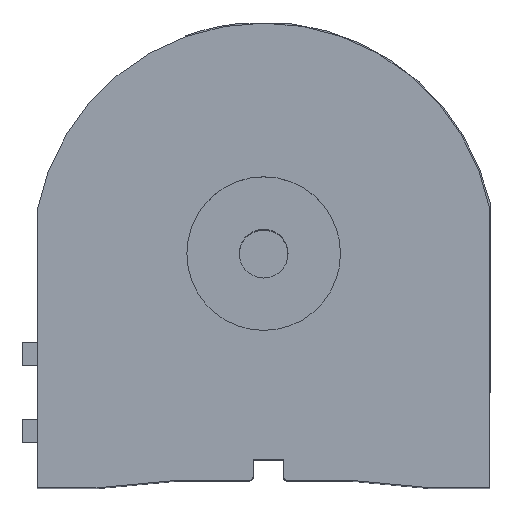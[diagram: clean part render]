
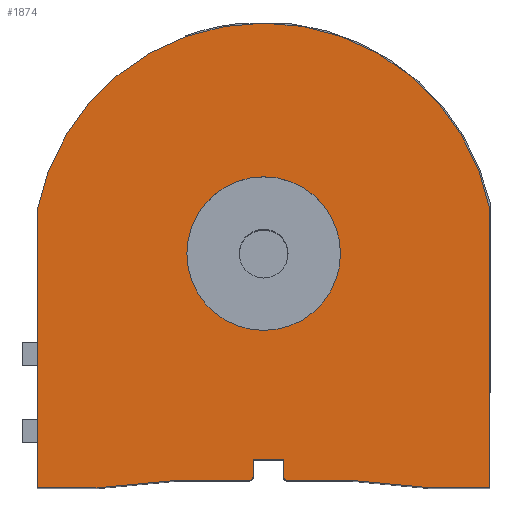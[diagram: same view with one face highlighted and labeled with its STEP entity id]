
A CAD part, top view. The second image highlights one B-rep face of the part: STEP entity #1874.
In plain terms, the highlighted planar face has unit normal (0, 0, 1).
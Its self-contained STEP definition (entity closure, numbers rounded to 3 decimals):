
#7 = CARTESIAN_POINT ( 'NONE',  ( -22.5, -59., 80. ) ) ;
#67 = ORIENTED_EDGE ( 'NONE', *, *, #3143, .F. ) ;
#74 = LINE ( 'NONE', #588, #1202 ) ;
#77 = ORIENTED_EDGE ( 'NONE', *, *, #887, .T. ) ;
#78 = LINE ( 'NONE', #2872, #2936 ) ;
#91 = EDGE_CURVE ( 'NONE', #2361, #855, #78, .T. ) ;
#120 = VERTEX_POINT ( 'NONE', #1077 ) ;
#165 = DIRECTION ( 'NONE',  ( 0., 0., 1. ) ) ;
#188 = LINE ( 'NONE', #1919, #3088 ) ;
#200 = FACE_OUTER_BOUND ( 'NONE', #2185, .T. ) ;
#226 = CARTESIAN_POINT ( 'NONE',  ( 5.083, -58., 80. ) ) ;
#251 = DIRECTION ( 'NONE',  ( -1., 0., 0. ) ) ;
#319 = VERTEX_POINT ( 'NONE', #458 ) ;
#347 = VECTOR ( 'NONE', #2061, 1000. ) ;
#356 = EDGE_CURVE ( 'NONE', #688, #815, #2359, .T. ) ;
#370 = CARTESIAN_POINT ( 'NONE',  ( -43.909, -61., 80. ) ) ;
#433 = EDGE_CURVE ( 'NONE', #1744, #2437, #3101, .T. ) ;
#435 = LINE ( 'NONE', #1690, #1250 ) ;
#446 = EDGE_CURVE ( 'NONE', #815, #3142, #2324, .T. ) ;
#458 = CARTESIAN_POINT ( 'NONE',  ( -3.75, -59., 80. ) ) ;
#480 = EDGE_LOOP ( 'NONE', ( #2577, #3135 ) ) ;
#489 = EDGE_CURVE ( 'NONE', #2361, #910, #1838, .T. ) ;
#490 = CARTESIAN_POINT ( 'NONE',  ( 0., 0., 80. ) ) ;
#495 = VERTEX_POINT ( 'NONE', #574 ) ;
#513 = EDGE_CURVE ( 'NONE', #1744, #714, #2102, .T. ) ;
#517 = EDGE_CURVE ( 'NONE', #855, #1277, #74, .T. ) ;
#518 = CIRCLE ( 'NONE', #3257, 20. ) ;
#574 = CARTESIAN_POINT ( 'NONE',  ( -20., 0., 80. ) ) ;
#588 = CARTESIAN_POINT ( 'NONE',  ( 5.083, -53.5, 80. ) ) ;
#611 = CIRCLE ( 'NONE', #2447, 20. ) ;
#667 = LINE ( 'NONE', #1197, #1941 ) ;
#688 = VERTEX_POINT ( 'NONE', #3011 ) ;
#714 = VERTEX_POINT ( 'NONE', #1204 ) ;
#741 = DIRECTION ( 'NONE',  ( 0., 0., 1. ) ) ;
#778 = VECTOR ( 'NONE', #1339, 1000. ) ;
#788 = ORIENTED_EDGE ( 'NONE', *, *, #489, .T. ) ;
#794 = EDGE_CURVE ( 'NONE', #2437, #688, #1452, .T. ) ;
#808 = LINE ( 'NONE', #1074, #2657 ) ;
#815 = VERTEX_POINT ( 'NONE', #3045 ) ;
#817 = CIRCLE ( 'NONE', #1404, 1. ) ;
#822 = CARTESIAN_POINT ( 'NONE',  ( -3.75, -58., 80. ) ) ;
#844 = CARTESIAN_POINT ( 'NONE',  ( -58.909, -61., 80. ) ) ;
#855 = VERTEX_POINT ( 'NONE', #2562 ) ;
#887 = EDGE_CURVE ( 'NONE', #319, #3008, #817, .T. ) ;
#910 = VERTEX_POINT ( 'NONE', #2580 ) ;
#1051 = CARTESIAN_POINT ( 'NONE',  ( -58.909, -61., 80. ) ) ;
#1074 = CARTESIAN_POINT ( 'NONE',  ( 58.909, -61., 80. ) ) ;
#1077 = CARTESIAN_POINT ( 'NONE',  ( 20., 0., 80. ) ) ;
#1078 = CARTESIAN_POINT ( 'NONE',  ( -2.75, -53.5, 80. ) ) ;
#1090 = AXIS2_PLACEMENT_3D ( 'NONE', #3216, #1494, #251 ) ;
#1092 = DIRECTION ( 'NONE',  ( -1., 0., 0. ) ) ;
#1179 = ORIENTED_EDGE ( 'NONE', *, *, #2942, .F. ) ;
#1197 = CARTESIAN_POINT ( 'NONE',  ( 22.5, -59., 80. ) ) ;
#1202 = VECTOR ( 'NONE', #1092, 1000. ) ;
#1204 = CARTESIAN_POINT ( 'NONE',  ( 22.5, -59., 80. ) ) ;
#1216 = ORIENTED_EDGE ( 'NONE', *, *, #91, .F. ) ;
#1240 = PLANE ( 'NONE',  #1090 ) ;
#1250 = VECTOR ( 'NONE', #2176, 1000. ) ;
#1256 = VECTOR ( 'NONE', #2119, 1000. ) ;
#1277 = VERTEX_POINT ( 'NONE', #1078 ) ;
#1280 = DIRECTION ( 'NONE',  ( 0., 0., 1. ) ) ;
#1339 = DIRECTION ( 'NONE',  ( -0.996, 0.093, 0. ) ) ;
#1404 = AXIS2_PLACEMENT_3D ( 'NONE', #822, #2810, #2596 ) ;
#1447 = DIRECTION ( 'NONE',  ( -1., 0., 0. ) ) ;
#1452 = LINE ( 'NONE', #2445, #2630 ) ;
#1494 = DIRECTION ( 'NONE',  ( 0., 0., -1. ) ) ;
#1612 = DIRECTION ( 'NONE',  ( 0., 1., 0. ) ) ;
#1636 = VECTOR ( 'NONE', #2067, 1000. ) ;
#1661 = EDGE_CURVE ( 'NONE', #3142, #1814, #808, .T. ) ;
#1688 = AXIS2_PLACEMENT_3D ( 'NONE', #490, #741, #2697 ) ;
#1690 = CARTESIAN_POINT ( 'NONE',  ( -2.75, -53.5, 80. ) ) ;
#1736 = CARTESIAN_POINT ( 'NONE',  ( 0., 0., 80. ) ) ;
#1744 = VERTEX_POINT ( 'NONE', #2656 ) ;
#1787 = AXIS2_PLACEMENT_3D ( 'NONE', #2835, #2338, #2049 ) ;
#1813 = EDGE_CURVE ( 'NONE', #495, #120, #518, .T. ) ;
#1814 = VERTEX_POINT ( 'NONE', #2435 ) ;
#1838 = CIRCLE ( 'NONE', #1787, 1. ) ;
#1874 = ADVANCED_FACE ( 'NONE', ( #1986, #200 ), #1240, .F. ) ;
#1919 = CARTESIAN_POINT ( 'NONE',  ( 22.5, -59., 80. ) ) ;
#1926 = ORIENTED_EDGE ( 'NONE', *, *, #794, .T. ) ;
#1941 = VECTOR ( 'NONE', #1447, 1000. ) ;
#1950 = DIRECTION ( 'NONE',  ( -1., 0., 0. ) ) ;
#1986 = FACE_BOUND ( 'NONE', #480, .T. ) ;
#1995 = CARTESIAN_POINT ( 'NONE',  ( -2.75, -58., 80. ) ) ;
#2049 = DIRECTION ( 'NONE',  ( -1., 0., 0. ) ) ;
#2061 = DIRECTION ( 'NONE',  ( -0.996, -0.093, 0. ) ) ;
#2067 = DIRECTION ( 'NONE',  ( 1., 0., 0. ) ) ;
#2075 = ORIENTED_EDGE ( 'NONE', *, *, #446, .T. ) ;
#2102 = LINE ( 'NONE', #2783, #778 ) ;
#2119 = DIRECTION ( 'NONE',  ( 0., -1., 0. ) ) ;
#2127 = LINE ( 'NONE', #370, #347 ) ;
#2176 = DIRECTION ( 'NONE',  ( 0., -1., 0. ) ) ;
#2185 = EDGE_LOOP ( 'NONE', ( #1216, #788, #3255, #2742, #2579, #1926, #2369, #2075, #2870, #67, #2809, #77, #1179, #2267 ) ) ;
#2267 = ORIENTED_EDGE ( 'NONE', *, *, #517, .F. ) ;
#2273 = CARTESIAN_POINT ( 'NONE',  ( 58.909, -61., 80. ) ) ;
#2324 = LINE ( 'NONE', #844, #1256 ) ;
#2338 = DIRECTION ( 'NONE',  ( 0., 0., 1. ) ) ;
#2359 = CIRCLE ( 'NONE', #1688, 60. ) ;
#2361 = VERTEX_POINT ( 'NONE', #226 ) ;
#2369 = ORIENTED_EDGE ( 'NONE', *, *, #356, .T. ) ;
#2422 = CARTESIAN_POINT ( 'NONE',  ( 0., 0., 80. ) ) ;
#2435 = CARTESIAN_POINT ( 'NONE',  ( -43.909, -61., 80. ) ) ;
#2437 = VERTEX_POINT ( 'NONE', #2273 ) ;
#2445 = CARTESIAN_POINT ( 'NONE',  ( 58.909, -61., 80. ) ) ;
#2447 = AXIS2_PLACEMENT_3D ( 'NONE', #1736, #1280, #2726 ) ;
#2535 = VERTEX_POINT ( 'NONE', #7 ) ;
#2562 = CARTESIAN_POINT ( 'NONE',  ( 5.083, -53.5, 80. ) ) ;
#2577 = ORIENTED_EDGE ( 'NONE', *, *, #3072, .F. ) ;
#2579 = ORIENTED_EDGE ( 'NONE', *, *, #433, .T. ) ;
#2580 = CARTESIAN_POINT ( 'NONE',  ( 6.083, -59., 80. ) ) ;
#2583 = CARTESIAN_POINT ( 'NONE',  ( 58.909, -61., 80. ) ) ;
#2596 = DIRECTION ( 'NONE',  ( -1., 0., 0. ) ) ;
#2630 = VECTOR ( 'NONE', #2710, 1000. ) ;
#2656 = CARTESIAN_POINT ( 'NONE',  ( 43.909, -61., 80. ) ) ;
#2657 = VECTOR ( 'NONE', #2836, 1000. ) ;
#2697 = DIRECTION ( 'NONE',  ( -1., 0., 0. ) ) ;
#2710 = DIRECTION ( 'NONE',  ( 0., 1., 0. ) ) ;
#2726 = DIRECTION ( 'NONE',  ( 1., 0., 0. ) ) ;
#2742 = ORIENTED_EDGE ( 'NONE', *, *, #513, .F. ) ;
#2783 = CARTESIAN_POINT ( 'NONE',  ( 43.909, -61., 80. ) ) ;
#2809 = ORIENTED_EDGE ( 'NONE', *, *, #3259, .F. ) ;
#2810 = DIRECTION ( 'NONE',  ( 0., 0., 1. ) ) ;
#2835 = CARTESIAN_POINT ( 'NONE',  ( 6.083, -58., 80. ) ) ;
#2836 = DIRECTION ( 'NONE',  ( 1., 0., 0. ) ) ;
#2870 = ORIENTED_EDGE ( 'NONE', *, *, #1661, .T. ) ;
#2872 = CARTESIAN_POINT ( 'NONE',  ( 5.083, -66.165, 80. ) ) ;
#2915 = EDGE_CURVE ( 'NONE', #714, #910, #188, .T. ) ;
#2936 = VECTOR ( 'NONE', #1612, 1000. ) ;
#2942 = EDGE_CURVE ( 'NONE', #1277, #3008, #435, .T. ) ;
#3008 = VERTEX_POINT ( 'NONE', #1995 ) ;
#3011 = CARTESIAN_POINT ( 'NONE',  ( 58.909, 11.39, 80. ) ) ;
#3045 = CARTESIAN_POINT ( 'NONE',  ( -58.909, 11.39, 80. ) ) ;
#3072 = EDGE_CURVE ( 'NONE', #120, #495, #611, .T. ) ;
#3088 = VECTOR ( 'NONE', #1950, 1000. ) ;
#3101 = LINE ( 'NONE', #2583, #1636 ) ;
#3135 = ORIENTED_EDGE ( 'NONE', *, *, #1813, .F. ) ;
#3142 = VERTEX_POINT ( 'NONE', #1051 ) ;
#3143 = EDGE_CURVE ( 'NONE', #2535, #1814, #2127, .T. ) ;
#3202 = DIRECTION ( 'NONE',  ( 1., 0., 0. ) ) ;
#3216 = CARTESIAN_POINT ( 'NONE',  ( 0., 0., 80. ) ) ;
#3255 = ORIENTED_EDGE ( 'NONE', *, *, #2915, .F. ) ;
#3257 = AXIS2_PLACEMENT_3D ( 'NONE', #2422, #165, #3202 ) ;
#3259 = EDGE_CURVE ( 'NONE', #319, #2535, #667, .T. ) ;
